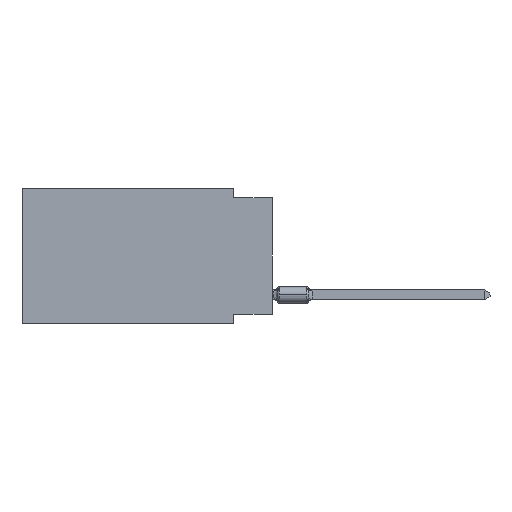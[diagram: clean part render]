
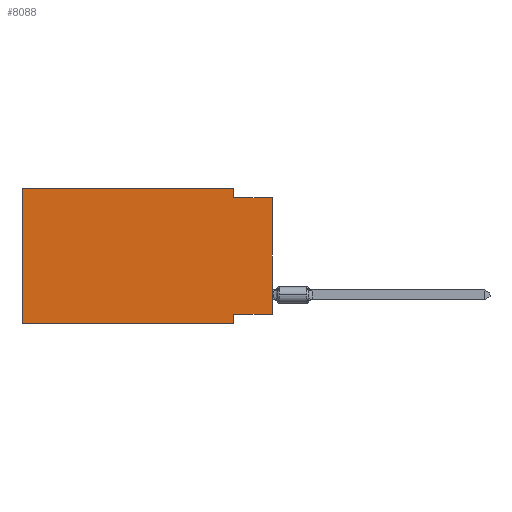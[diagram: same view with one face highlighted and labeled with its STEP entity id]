
A CAD part, left-side view. The second image highlights one B-rep face of the part: STEP entity #8088.
In plain terms, the highlighted planar face has unit normal (-1, 0, 0).
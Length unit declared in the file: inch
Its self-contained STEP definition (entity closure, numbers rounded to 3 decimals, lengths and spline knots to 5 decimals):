
#312 = EDGE_CURVE ( 'NONE', #15551, #5788, #9549, .T. ) ;
#502 = CARTESIAN_POINT ( 'NONE',  ( 0., 0., -0.025 ) ) ;
#524 = CARTESIAN_POINT ( 'NONE',  ( 0., 0., -0.025 ) ) ;
#650 = FACE_OUTER_BOUND ( 'NONE', #3017, .T. ) ;
#951 = EDGE_CURVE ( 'NONE', #6625, #6915, #7528, .T. ) ;
#1101 = EDGE_CURVE ( 'NONE', #5394, #5788, #8192, .T. ) ;
#1181 = VECTOR ( 'NONE', #3258, 39.37008 ) ;
#1843 = EDGE_CURVE ( 'NONE', #3296, #11362, #2712, .T. ) ;
#1990 = EDGE_CURVE ( 'NONE', #11362, #15551, #4450, .T. ) ;
#2273 = VECTOR ( 'NONE', #9378, 39.37008 ) ;
#2556 = VERTEX_POINT ( 'NONE', #6165 ) ;
#2712 = LINE ( 'NONE', #6485, #14881 ) ;
#2878 = VECTOR ( 'NONE', #4555, 39.37008 ) ;
#3017 = EDGE_LOOP ( 'NONE', ( #6444, #11480, #12674, #3377, #13649, #11731, #9319, #5559 ) ) ;
#3258 = DIRECTION ( 'NONE',  ( 0., -1., 0. ) ) ;
#3296 = VERTEX_POINT ( 'NONE', #4613 ) ;
#3355 = LINE ( 'NONE', #13486, #10473 ) ;
#3377 = ORIENTED_EDGE ( 'NONE', *, *, #1843, .F. ) ;
#3847 = CARTESIAN_POINT ( 'NONE',  ( 0., 0.1, 0. ) ) ;
#4227 = CARTESIAN_POINT ( 'NONE',  ( 0., 0.645, -0.35 ) ) ;
#4247 = DIRECTION ( 'NONE',  ( 0., 0., -1. ) ) ;
#4318 = CARTESIAN_POINT ( 'NONE',  ( 0., 0.1, -0.35 ) ) ;
#4438 = EDGE_CURVE ( 'NONE', #2556, #6915, #6738, .T. ) ;
#4450 = LINE ( 'NONE', #7050, #10343 ) ;
#4555 = DIRECTION ( 'NONE',  ( 0., 1., 0. ) ) ;
#4613 = CARTESIAN_POINT ( 'NONE',  ( 0., 0.645, 0. ) ) ;
#4867 = CARTESIAN_POINT ( 'NONE',  ( 0., 0.1, -0.025 ) ) ;
#4901 = VECTOR ( 'NONE', #11843, 39.37008 ) ;
#5394 = VERTEX_POINT ( 'NONE', #14138 ) ;
#5538 = EDGE_CURVE ( 'NONE', #5394, #6625, #16297, .T. ) ;
#5559 = ORIENTED_EDGE ( 'NONE', *, *, #5538, .F. ) ;
#5745 = CARTESIAN_POINT ( 'NONE',  ( 0., 0.645, 0. ) ) ;
#5788 = VERTEX_POINT ( 'NONE', #524 ) ;
#6165 = CARTESIAN_POINT ( 'NONE',  ( 0., 0.645, -0.35 ) ) ;
#6444 = ORIENTED_EDGE ( 'NONE', *, *, #1101, .T. ) ;
#6485 = CARTESIAN_POINT ( 'NONE',  ( 0., 0.645, 0. ) ) ;
#6625 = VERTEX_POINT ( 'NONE', #8184 ) ;
#6738 = LINE ( 'NONE', #4227, #4901 ) ;
#6915 = VERTEX_POINT ( 'NONE', #4318 ) ;
#7050 = CARTESIAN_POINT ( 'NONE',  ( 0., 0.1, 0. ) ) ;
#7528 = LINE ( 'NONE', #15318, #14590 ) ;
#7720 = AXIS2_PLACEMENT_3D ( 'NONE', #5745, #12200, #4247 ) ;
#7991 = DIRECTION ( 'NONE',  ( 0., -1., 0. ) ) ;
#8088 = ADVANCED_FACE ( 'NONE', ( #650 ), #10624, .F. ) ;
#8184 = CARTESIAN_POINT ( 'NONE',  ( 0., 0.1, -0.325 ) ) ;
#8192 = LINE ( 'NONE', #14319, #2273 ) ;
#8239 = DIRECTION ( 'NONE',  ( 0., 0., -1. ) ) ;
#8598 = CARTESIAN_POINT ( 'NONE',  ( 0., 0., -0.325 ) ) ;
#9319 = ORIENTED_EDGE ( 'NONE', *, *, #951, .F. ) ;
#9378 = DIRECTION ( 'NONE',  ( 0., 0., 1. ) ) ;
#9549 = LINE ( 'NONE', #502, #1181 ) ;
#10343 = VECTOR ( 'NONE', #8239, 39.37008 ) ;
#10473 = VECTOR ( 'NONE', #12309, 39.37008 ) ;
#10624 = PLANE ( 'NONE',  #7720 ) ;
#11362 = VERTEX_POINT ( 'NONE', #3847 ) ;
#11480 = ORIENTED_EDGE ( 'NONE', *, *, #312, .F. ) ;
#11731 = ORIENTED_EDGE ( 'NONE', *, *, #4438, .T. ) ;
#11843 = DIRECTION ( 'NONE',  ( 0., -1., 0. ) ) ;
#12200 = DIRECTION ( 'NONE',  ( 1., 0., 0. ) ) ;
#12309 = DIRECTION ( 'NONE',  ( 0., 0., 1. ) ) ;
#12452 = EDGE_CURVE ( 'NONE', #2556, #3296, #3355, .T. ) ;
#12646 = DIRECTION ( 'NONE',  ( 0., 0., -1. ) ) ;
#12674 = ORIENTED_EDGE ( 'NONE', *, *, #1990, .F. ) ;
#13486 = CARTESIAN_POINT ( 'NONE',  ( 0., 0.645, 0. ) ) ;
#13649 = ORIENTED_EDGE ( 'NONE', *, *, #12452, .F. ) ;
#14138 = CARTESIAN_POINT ( 'NONE',  ( 0., 0., -0.325 ) ) ;
#14319 = CARTESIAN_POINT ( 'NONE',  ( 0., 0., 0. ) ) ;
#14590 = VECTOR ( 'NONE', #12646, 39.37008 ) ;
#14881 = VECTOR ( 'NONE', #7991, 39.37008 ) ;
#15318 = CARTESIAN_POINT ( 'NONE',  ( 0., 0.1, -0.35 ) ) ;
#15551 = VERTEX_POINT ( 'NONE', #4867 ) ;
#16297 = LINE ( 'NONE', #8598, #2878 ) ;
